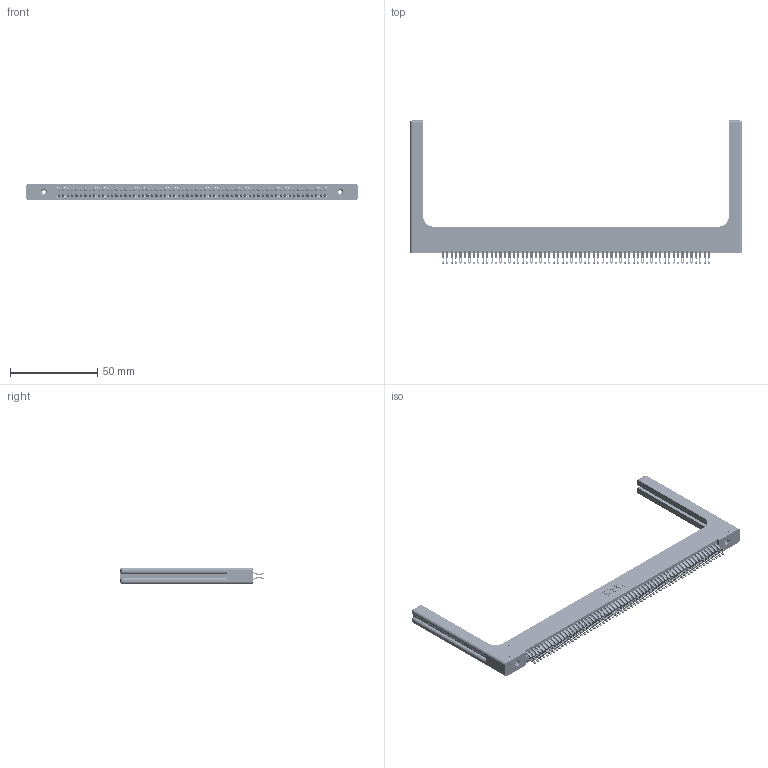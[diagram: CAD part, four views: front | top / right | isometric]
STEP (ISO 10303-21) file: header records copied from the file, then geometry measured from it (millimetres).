
FILE_DESCRIPTION (( 'STEP AP203' ), '1' );
FILE_NAME ('395-122-555-258.STEP', '2019-10-28T08:46:24', ( '' ), ( '' ), 'SwSTEP 2.0', 'SolidWorks 2016', '' );
FILE_SCHEMA (( 'CONFIG_CONTROL_DESIGN' ));
Length unit declared in the file: inch
Products named in the file (5): 345 Part_Flush Mounting Lugs - 0.156 Dia-TH; 345-292-001_555 Tail; 345-250-001_345-250-001-102; 345-220-058_345-220-058; 395-122-555-258
Assembly tree (127 placements, depth 2):
  395-122-555-258
    345 Part_Flush Mounting Lugs - 0.156 Dia-TH
    345-292-001_555 Tail  x122
    345-250-001_345-250-001-102  x2
    345-220-058_345-220-058  x2
Bounding box: 189.97 x 82.09 x 9.4 mm (x, y, z)
Volume: 27458.9 mm3; surface area: 34718.9 mm2
Topology: 127 solids, 127 shells, 7214 faces, 22601 edges, 15046 vertices
Faces by surface type: plane 4010, cylinder 3144, bspline 36, cone 12, sphere 8, torus 4
Entity records: 50812 total; most frequent: CARTESIAN_POINT 9527, ORIENTED_EDGE 8228, DIRECTION 7278, EDGE_CURVE 4114, LINE 3626, VECTOR 3626, VERTEX_POINT 2734, AXIS2_PLACEMENT_3D 1826
